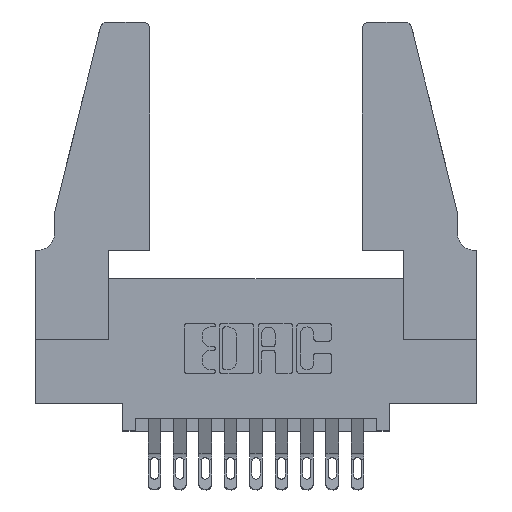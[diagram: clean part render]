
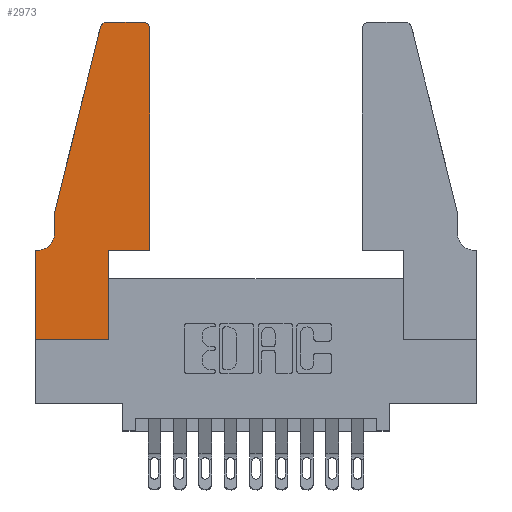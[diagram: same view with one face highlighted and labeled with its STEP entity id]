
A CAD part, top view. The second image highlights one B-rep face of the part: STEP entity #2973.
In plain terms, the highlighted planar face has unit normal (0, 0, 1).
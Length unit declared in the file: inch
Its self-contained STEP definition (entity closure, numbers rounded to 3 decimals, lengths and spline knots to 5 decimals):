
#202 = DIRECTION ( 'NONE',  ( 1., 0., 0. ) ) ;
#351 = LINE ( 'NONE', #5335, #6627 ) ;
#543 = AXIS2_PLACEMENT_3D ( 'NONE', #3337, #10949, #4447 ) ;
#892 = CARTESIAN_POINT ( 'NONE',  ( 0.2865, 0.35, 0.37 ) ) ;
#897 = EDGE_CURVE ( 'NONE', #2040, #6068, #8879, .T. ) ;
#974 = DIRECTION ( 'NONE',  ( 0., -1., 0. ) ) ;
#998 = EDGE_CURVE ( 'NONE', #10767, #2843, #10743, .T. ) ;
#1060 = VERTEX_POINT ( 'NONE', #5484 ) ;
#1141 = ORIENTED_EDGE ( 'NONE', *, *, #4176, .T. ) ;
#1187 = EDGE_CURVE ( 'NONE', #10762, #2040, #5500, .T. ) ;
#1239 = CIRCLE ( 'NONE', #5136, 0.07 ) ;
#1357 = VECTOR ( 'NONE', #10777, 39.37008 ) ;
#1471 = CARTESIAN_POINT ( 'NONE',  ( 0.2605, 1.25, 0.37 ) ) ;
#1487 = CARTESIAN_POINT ( 'NONE',  ( 0., 0., 0.37 ) ) ;
#1930 = VERTEX_POINT ( 'NONE', #7739 ) ;
#2029 = VECTOR ( 'NONE', #202, 39.37008 ) ;
#2040 = VERTEX_POINT ( 'NONE', #14069 ) ;
#2069 = CARTESIAN_POINT ( 'NONE',  ( 0.25487, 1.22718, 0.37 ) ) ;
#2271 = CARTESIAN_POINT ( 'NONE',  ( 0., 0.35, 0.37 ) ) ;
#2473 = EDGE_CURVE ( 'NONE', #11794, #1060, #7338, .T. ) ;
#2518 = ORIENTED_EDGE ( 'NONE', *, *, #897, .T. ) ;
#2616 = DIRECTION ( 'NONE',  ( -1., 0., 0. ) ) ;
#2643 = CARTESIAN_POINT ( 'NONE',  ( 0.0755, 0.5, 0.37 ) ) ;
#2666 = EDGE_CURVE ( 'NONE', #2843, #13785, #7841, .T. ) ;
#2824 = VERTEX_POINT ( 'NONE', #4739 ) ;
#2843 = VERTEX_POINT ( 'NONE', #6131 ) ;
#2973 = ADVANCED_FACE ( 'NONE', ( #4789 ), #13610, .T. ) ;
#3059 = CARTESIAN_POINT ( 'NONE',  ( 0., 0., 0.37 ) ) ;
#3064 = VECTOR ( 'NONE', #7884, 39.37008 ) ;
#3337 = CARTESIAN_POINT ( 'NONE',  ( 0.284, 1.22, 0.37 ) ) ;
#3347 = EDGE_CURVE ( 'NONE', #6068, #10767, #1239, .T. ) ;
#3456 = ORIENTED_EDGE ( 'NONE', *, *, #5309, .T. ) ;
#3583 = ORIENTED_EDGE ( 'NONE', *, *, #11352, .T. ) ;
#4048 = ORIENTED_EDGE ( 'NONE', *, *, #4063, .T. ) ;
#4063 = EDGE_CURVE ( 'NONE', #13785, #8325, #351, .T. ) ;
#4176 = EDGE_CURVE ( 'NONE', #10598, #10762, #4227, .T. ) ;
#4227 = CIRCLE ( 'NONE', #543, 0.03 ) ;
#4238 = ORIENTED_EDGE ( 'NONE', *, *, #2666, .T. ) ;
#4275 = CARTESIAN_POINT ( 'NONE',  ( 0.4505, 0.35, 0.37 ) ) ;
#4346 = CARTESIAN_POINT ( 'NONE',  ( 0.0055, 0.35, 0.37 ) ) ;
#4363 = LINE ( 'NONE', #4275, #1357 ) ;
#4447 = DIRECTION ( 'NONE',  ( 1., 0., 0. ) ) ;
#4668 = AXIS2_PLACEMENT_3D ( 'NONE', #2271, #13514, #13500 ) ;
#4739 = CARTESIAN_POINT ( 'NONE',  ( 0.2865, 0.35, 0.37 ) ) ;
#4789 = FACE_OUTER_BOUND ( 'NONE', #13222, .T. ) ;
#4994 = VECTOR ( 'NONE', #12442, 39.37008 ) ;
#5136 = AXIS2_PLACEMENT_3D ( 'NONE', #10803, #10709, #8248 ) ;
#5309 = EDGE_CURVE ( 'NONE', #1930, #11794, #4363, .T. ) ;
#5335 = CARTESIAN_POINT ( 'NONE',  ( 0., 0., 0.37 ) ) ;
#5484 = CARTESIAN_POINT ( 'NONE',  ( 0.4205, 1.25, 0.37 ) ) ;
#5500 = LINE ( 'NONE', #14020, #8713 ) ;
#6005 = DIRECTION ( 'NONE',  ( 1., 0., 0. ) ) ;
#6008 = DIRECTION ( 'NONE',  ( 0., 0., 1. ) ) ;
#6016 = CARTESIAN_POINT ( 'NONE',  ( 0.4205, 1.22, 0.37 ) ) ;
#6068 = VERTEX_POINT ( 'NONE', #6693 ) ;
#6131 = CARTESIAN_POINT ( 'NONE',  ( 0., 0.35, 0.37 ) ) ;
#6166 = EDGE_CURVE ( 'NONE', #2824, #1930, #7905, .T. ) ;
#6216 = CARTESIAN_POINT ( 'NONE',  ( 0.284, 1.25, 0.37 ) ) ;
#6272 = EDGE_CURVE ( 'NONE', #1060, #10598, #6898, .T. ) ;
#6627 = VECTOR ( 'NONE', #11781, 39.37008 ) ;
#6693 = CARTESIAN_POINT ( 'NONE',  ( 0.0755, 0.42, 0.37 ) ) ;
#6791 = CARTESIAN_POINT ( 'NONE',  ( 0.2865, 0., 0.37 ) ) ;
#6835 = CARTESIAN_POINT ( 'NONE',  ( 0.4505, 0.35, 0.37 ) ) ;
#6898 = LINE ( 'NONE', #1471, #12274 ) ;
#7338 = CIRCLE ( 'NONE', #8846, 0.03 ) ;
#7739 = CARTESIAN_POINT ( 'NONE',  ( 0.4505, 0.35, 0.37 ) ) ;
#7841 = LINE ( 'NONE', #1487, #10381 ) ;
#7884 = DIRECTION ( 'NONE',  ( 0., -1., 0. ) ) ;
#7905 = LINE ( 'NONE', #6835, #2029 ) ;
#8194 = ORIENTED_EDGE ( 'NONE', *, *, #2473, .T. ) ;
#8248 = DIRECTION ( 'NONE',  ( -1., 0., 0. ) ) ;
#8325 = VERTEX_POINT ( 'NONE', #6791 ) ;
#8606 = DIRECTION ( 'NONE',  ( 0., 1., 0. ) ) ;
#8713 = VECTOR ( 'NONE', #13426, 39.37008 ) ;
#8815 = LINE ( 'NONE', #892, #12014 ) ;
#8846 = AXIS2_PLACEMENT_3D ( 'NONE', #6016, #6008, #6005 ) ;
#8858 = ORIENTED_EDGE ( 'NONE', *, *, #6166, .T. ) ;
#8879 = LINE ( 'NONE', #2643, #3064 ) ;
#9270 = ORIENTED_EDGE ( 'NONE', *, *, #3347, .T. ) ;
#9564 = ORIENTED_EDGE ( 'NONE', *, *, #6272, .T. ) ;
#9961 = ORIENTED_EDGE ( 'NONE', *, *, #998, .T. ) ;
#10381 = VECTOR ( 'NONE', #974, 39.37008 ) ;
#10398 = CARTESIAN_POINT ( 'NONE',  ( 0.4505, 1.22, 0.37 ) ) ;
#10598 = VERTEX_POINT ( 'NONE', #6216 ) ;
#10709 = DIRECTION ( 'NONE',  ( 0., 0., -1. ) ) ;
#10743 = LINE ( 'NONE', #12473, #4994 ) ;
#10762 = VERTEX_POINT ( 'NONE', #2069 ) ;
#10767 = VERTEX_POINT ( 'NONE', #4346 ) ;
#10777 = DIRECTION ( 'NONE',  ( 0., 1., 0. ) ) ;
#10803 = CARTESIAN_POINT ( 'NONE',  ( 0.0055, 0.42, 0.37 ) ) ;
#10949 = DIRECTION ( 'NONE',  ( 0., 0., 1. ) ) ;
#11112 = ORIENTED_EDGE ( 'NONE', *, *, #1187, .T. ) ;
#11352 = EDGE_CURVE ( 'NONE', #8325, #2824, #8815, .T. ) ;
#11781 = DIRECTION ( 'NONE',  ( 1., 0., 0. ) ) ;
#11794 = VERTEX_POINT ( 'NONE', #10398 ) ;
#12014 = VECTOR ( 'NONE', #8606, 39.37008 ) ;
#12274 = VECTOR ( 'NONE', #2616, 39.37008 ) ;
#12442 = DIRECTION ( 'NONE',  ( -1., 0., 0. ) ) ;
#12473 = CARTESIAN_POINT ( 'NONE',  ( 0.0755, 0.35, 0.37 ) ) ;
#13222 = EDGE_LOOP ( 'NONE', ( #9564, #1141, #11112, #2518, #9270, #9961, #4238, #4048, #3583, #8858, #3456, #8194 ) ) ;
#13426 = DIRECTION ( 'NONE',  ( -0.239, -0.971, 0. ) ) ;
#13500 = DIRECTION ( 'NONE',  ( 1., 0., 0. ) ) ;
#13514 = DIRECTION ( 'NONE',  ( 0., 0., 1. ) ) ;
#13610 = PLANE ( 'NONE',  #4668 ) ;
#13785 = VERTEX_POINT ( 'NONE', #3059 ) ;
#14020 = CARTESIAN_POINT ( 'NONE',  ( 0.0755, 0.5, 0.37 ) ) ;
#14069 = CARTESIAN_POINT ( 'NONE',  ( 0.0755, 0.5, 0.37 ) ) ;
